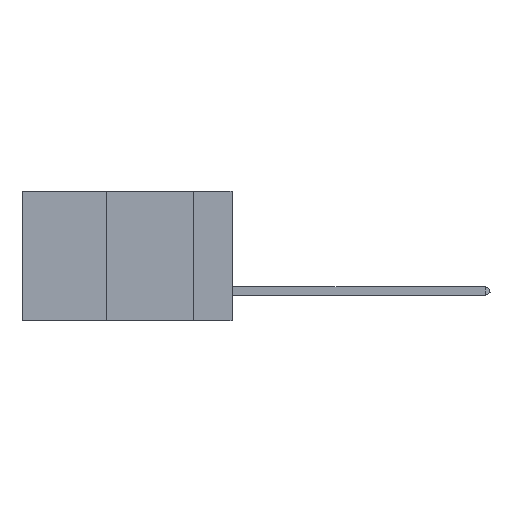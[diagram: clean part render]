
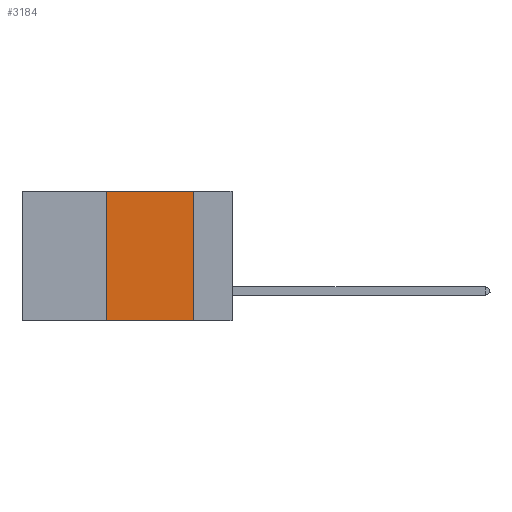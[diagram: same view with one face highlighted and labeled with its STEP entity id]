
A CAD part, left-side view. The second image highlights one B-rep face of the part: STEP entity #3184.
In plain terms, the highlighted planar face has unit normal (-1, 0, 0).
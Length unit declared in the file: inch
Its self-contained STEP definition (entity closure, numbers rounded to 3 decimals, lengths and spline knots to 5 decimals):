
#269 = VERTEX_POINT ( 'NONE', #2050 ) ;
#542 = EDGE_CURVE ( 'NONE', #9143, #3337, #3229, .T. ) ;
#578 = DIRECTION ( 'NONE',  ( 0., 0., -1. ) ) ;
#970 = VECTOR ( 'NONE', #1583, 39.37008 ) ;
#986 = CARTESIAN_POINT ( 'NONE',  ( 0., 0.36, 0. ) ) ;
#1330 = ORIENTED_EDGE ( 'NONE', *, *, #542, .F. ) ;
#1343 = ORIENTED_EDGE ( 'NONE', *, *, #8685, .F. ) ;
#1454 = CARTESIAN_POINT ( 'NONE',  ( 0., 0.36, -0.37 ) ) ;
#1583 = DIRECTION ( 'NONE',  ( 0., -1., 0. ) ) ;
#1912 = DIRECTION ( 'NONE',  ( 0., 0., 1. ) ) ;
#2050 = CARTESIAN_POINT ( 'NONE',  ( 0., 0.36, 0. ) ) ;
#3184 = ADVANCED_FACE ( 'NONE', ( #8948 ), #8432, .F. ) ;
#3229 = LINE ( 'NONE', #13039, #3900 ) ;
#3291 = DIRECTION ( 'NONE',  ( 0., 0., -1. ) ) ;
#3337 = VERTEX_POINT ( 'NONE', #8197 ) ;
#3900 = VECTOR ( 'NONE', #578, 39.37008 ) ;
#4157 = EDGE_LOOP ( 'NONE', ( #1330, #10778, #1343, #11681 ) ) ;
#4525 = CARTESIAN_POINT ( 'NONE',  ( 0., 0.6, 0. ) ) ;
#5141 = LINE ( 'NONE', #986, #12676 ) ;
#5851 = CARTESIAN_POINT ( 'NONE',  ( 0., 0.11, 0. ) ) ;
#5987 = AXIS2_PLACEMENT_3D ( 'NONE', #7321, #10620, #3291 ) ;
#6622 = EDGE_CURVE ( 'NONE', #269, #9143, #6872, .T. ) ;
#6872 = LINE ( 'NONE', #4525, #12305 ) ;
#7321 = CARTESIAN_POINT ( 'NONE',  ( 0., 0.6, 0. ) ) ;
#8197 = CARTESIAN_POINT ( 'NONE',  ( 0., 0.11, -0.37 ) ) ;
#8432 = PLANE ( 'NONE',  #5987 ) ;
#8685 = EDGE_CURVE ( 'NONE', #9282, #269, #5141, .T. ) ;
#8948 = FACE_OUTER_BOUND ( 'NONE', #4157, .T. ) ;
#9143 = VERTEX_POINT ( 'NONE', #5851 ) ;
#9282 = VERTEX_POINT ( 'NONE', #1454 ) ;
#10620 = DIRECTION ( 'NONE',  ( 1., 0., 0. ) ) ;
#10739 = EDGE_CURVE ( 'NONE', #9282, #3337, #12132, .T. ) ;
#10778 = ORIENTED_EDGE ( 'NONE', *, *, #6622, .F. ) ;
#10879 = CARTESIAN_POINT ( 'NONE',  ( 0., 0.6, -0.37 ) ) ;
#11681 = ORIENTED_EDGE ( 'NONE', *, *, #10739, .T. ) ;
#12132 = LINE ( 'NONE', #10879, #970 ) ;
#12305 = VECTOR ( 'NONE', #13022, 39.37008 ) ;
#12676 = VECTOR ( 'NONE', #1912, 39.37008 ) ;
#13022 = DIRECTION ( 'NONE',  ( 0., -1., 0. ) ) ;
#13039 = CARTESIAN_POINT ( 'NONE',  ( 0., 0.11, 0. ) ) ;
